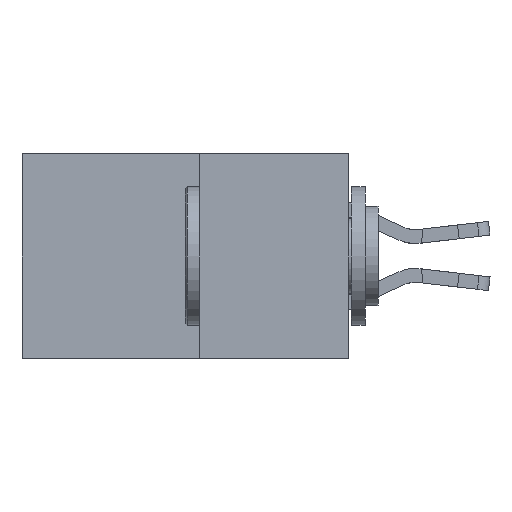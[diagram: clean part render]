
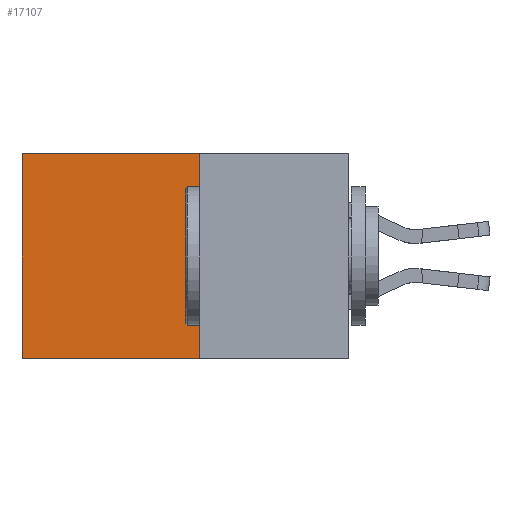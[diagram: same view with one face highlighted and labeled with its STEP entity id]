
A CAD part, left-side view. The second image highlights one B-rep face of the part: STEP entity #17107.
In plain terms, the highlighted planar face has unit normal (-1, 0, 0).
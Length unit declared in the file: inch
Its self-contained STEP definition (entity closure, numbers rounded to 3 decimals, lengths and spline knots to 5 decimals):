
#449 = VECTOR ( 'NONE', #14283, 39.37008 ) ;
#1567 = DIRECTION ( 'NONE',  ( 0., 1., 0. ) ) ;
#1709 = ORIENTED_EDGE ( 'NONE', *, *, #11737, .T. ) ;
#4238 = CARTESIAN_POINT ( 'NONE',  ( 0.277, 0.59, 0. ) ) ;
#5460 = PLANE ( 'NONE',  #18621 ) ;
#6897 = DIRECTION ( 'NONE',  ( 0., 0., -1. ) ) ;
#6911 = ORIENTED_EDGE ( 'NONE', *, *, #25175, .F. ) ;
#8022 = VECTOR ( 'NONE', #21464, 39.37008 ) ;
#8766 = ORIENTED_EDGE ( 'NONE', *, *, #19591, .F. ) ;
#9522 = DIRECTION ( 'NONE',  ( 0., 0., -1. ) ) ;
#10196 = CARTESIAN_POINT ( 'NONE',  ( 0.277, 0.59, -0.37 ) ) ;
#10347 = CARTESIAN_POINT ( 'NONE',  ( 0.277, 0.27, 0. ) ) ;
#11737 = EDGE_CURVE ( 'NONE', #16698, #19810, #15510, .T. ) ;
#12008 = EDGE_CURVE ( 'NONE', #19810, #12290, #19290, .T. ) ;
#12290 = VERTEX_POINT ( 'NONE', #10196 ) ;
#13521 = LINE ( 'NONE', #19417, #8022 ) ;
#13702 = CARTESIAN_POINT ( 'NONE',  ( 0.277, 0.27, -0.37 ) ) ;
#14283 = DIRECTION ( 'NONE',  ( 0., 1., 0. ) ) ;
#15510 = LINE ( 'NONE', #16279, #449 ) ;
#16279 = CARTESIAN_POINT ( 'NONE',  ( 0.277, 0.27, 0. ) ) ;
#16417 = EDGE_LOOP ( 'NONE', ( #19470, #8766, #6911, #1709 ) ) ;
#16695 = LINE ( 'NONE', #21905, #26176 ) ;
#16698 = VERTEX_POINT ( 'NONE', #10347 ) ;
#17107 = ADVANCED_FACE ( 'NONE', ( #20913 ), #5460, .F. ) ;
#17122 = VERTEX_POINT ( 'NONE', #13702 ) ;
#18621 = AXIS2_PLACEMENT_3D ( 'NONE', #19761, #21818, #9522 ) ;
#19290 = LINE ( 'NONE', #23253, #24675 ) ;
#19417 = CARTESIAN_POINT ( 'NONE',  ( 0.277, 0.27, -0.37 ) ) ;
#19470 = ORIENTED_EDGE ( 'NONE', *, *, #12008, .T. ) ;
#19591 = EDGE_CURVE ( 'NONE', #17122, #12290, #16695, .T. ) ;
#19761 = CARTESIAN_POINT ( 'NONE',  ( 0.277, 0.27, -0.37 ) ) ;
#19810 = VERTEX_POINT ( 'NONE', #4238 ) ;
#20913 = FACE_OUTER_BOUND ( 'NONE', #16417, .T. ) ;
#21464 = DIRECTION ( 'NONE',  ( 0., 0., -1. ) ) ;
#21818 = DIRECTION ( 'NONE',  ( 1., 0., 0. ) ) ;
#21905 = CARTESIAN_POINT ( 'NONE',  ( 0.277, 0.27, -0.37 ) ) ;
#23253 = CARTESIAN_POINT ( 'NONE',  ( 0.277, 0.59, -0.37 ) ) ;
#24675 = VECTOR ( 'NONE', #6897, 39.37008 ) ;
#25175 = EDGE_CURVE ( 'NONE', #16698, #17122, #13521, .T. ) ;
#26176 = VECTOR ( 'NONE', #1567, 39.37008 ) ;
